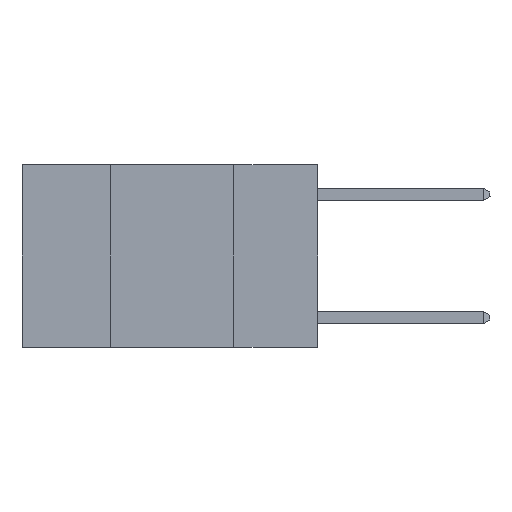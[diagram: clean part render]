
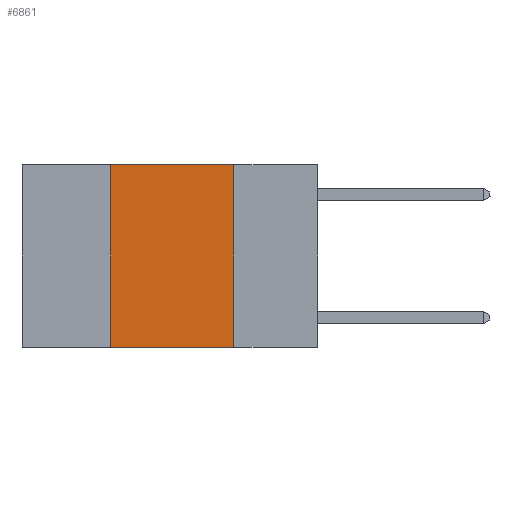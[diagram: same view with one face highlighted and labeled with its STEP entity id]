
A CAD part, left-side view. The second image highlights one B-rep face of the part: STEP entity #6861.
In plain terms, the highlighted planar face has unit normal (-1, 0, 0).
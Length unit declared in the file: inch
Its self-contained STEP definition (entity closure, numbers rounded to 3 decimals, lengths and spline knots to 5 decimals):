
#167 = ORIENTED_EDGE ( 'NONE', *, *, #17931, .F. ) ;
#2006 = CARTESIAN_POINT ( 'NONE',  ( 0., 0.17, 0. ) ) ;
#2495 = EDGE_LOOP ( 'NONE', ( #2739, #167, #16594, #9911 ) ) ;
#2739 = ORIENTED_EDGE ( 'NONE', *, *, #16047, .F. ) ;
#3010 = VECTOR ( 'NONE', #8284, 39.37008 ) ;
#3528 = VERTEX_POINT ( 'NONE', #9371 ) ;
#3551 = DIRECTION ( 'NONE',  ( 0., 0., -1. ) ) ;
#4289 = CARTESIAN_POINT ( 'NONE',  ( 0., 0.17, 0. ) ) ;
#4422 = PLANE ( 'NONE',  #5413 ) ;
#4463 = FACE_OUTER_BOUND ( 'NONE', #2495, .T. ) ;
#4871 = DIRECTION ( 'NONE',  ( 0., -1., 0. ) ) ;
#5413 = AXIS2_PLACEMENT_3D ( 'NONE', #13670, #5992, #16780 ) ;
#5992 = DIRECTION ( 'NONE',  ( 1., 0., 0. ) ) ;
#6861 = ADVANCED_FACE ( 'NONE', ( #4463 ), #4422, .F. ) ;
#7316 = CARTESIAN_POINT ( 'NONE',  ( 0., 0.17, -0.37 ) ) ;
#8060 = VECTOR ( 'NONE', #10501, 39.37008 ) ;
#8255 = VECTOR ( 'NONE', #3551, 39.37008 ) ;
#8284 = DIRECTION ( 'NONE',  ( 0., -1., 0. ) ) ;
#9371 = CARTESIAN_POINT ( 'NONE',  ( 0., 0.42, 0. ) ) ;
#9759 = VECTOR ( 'NONE', #4871, 39.37008 ) ;
#9911 = ORIENTED_EDGE ( 'NONE', *, *, #14575, .T. ) ;
#10501 = DIRECTION ( 'NONE',  ( 0., 0., 1. ) ) ;
#10931 = CARTESIAN_POINT ( 'NONE',  ( 0., 0.42, -0.37 ) ) ;
#11118 = CARTESIAN_POINT ( 'NONE',  ( 0., 0.6, -0.37 ) ) ;
#11337 = VERTEX_POINT ( 'NONE', #7316 ) ;
#12908 = VERTEX_POINT ( 'NONE', #10931 ) ;
#13670 = CARTESIAN_POINT ( 'NONE',  ( 0., 0.6, 0. ) ) ;
#14575 = EDGE_CURVE ( 'NONE', #12908, #11337, #18824, .T. ) ;
#14928 = EDGE_CURVE ( 'NONE', #12908, #3528, #19775, .T. ) ;
#14949 = VERTEX_POINT ( 'NONE', #4289 ) ;
#16047 = EDGE_CURVE ( 'NONE', #14949, #11337, #16398, .T. ) ;
#16398 = LINE ( 'NONE', #2006, #8255 ) ;
#16594 = ORIENTED_EDGE ( 'NONE', *, *, #14928, .F. ) ;
#16780 = DIRECTION ( 'NONE',  ( 0., 0., -1. ) ) ;
#17931 = EDGE_CURVE ( 'NONE', #3528, #14949, #19393, .T. ) ;
#18824 = LINE ( 'NONE', #11118, #9759 ) ;
#18956 = CARTESIAN_POINT ( 'NONE',  ( 0., 0.6, 0. ) ) ;
#19393 = LINE ( 'NONE', #18956, #3010 ) ;
#19619 = CARTESIAN_POINT ( 'NONE',  ( 0., 0.42, 0. ) ) ;
#19775 = LINE ( 'NONE', #19619, #8060 ) ;
